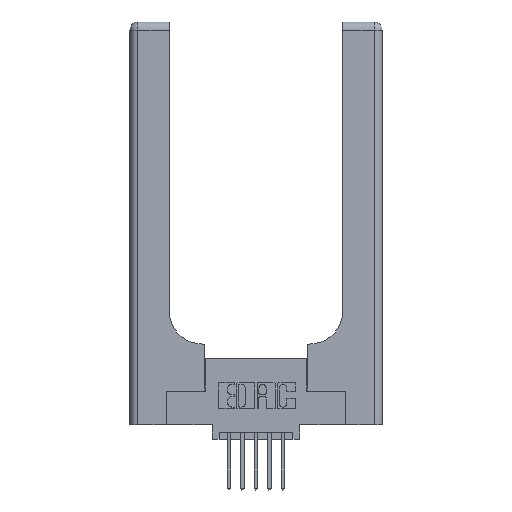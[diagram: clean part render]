
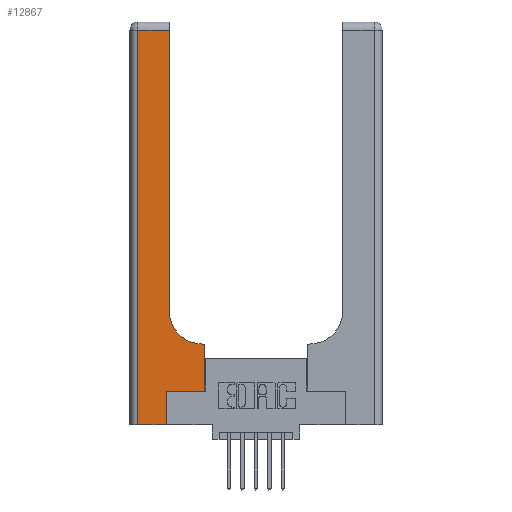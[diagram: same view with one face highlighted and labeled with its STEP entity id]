
A CAD part, top view. The second image highlights one B-rep face of the part: STEP entity #12867.
In plain terms, the highlighted planar face has unit normal (0, 0, 1).
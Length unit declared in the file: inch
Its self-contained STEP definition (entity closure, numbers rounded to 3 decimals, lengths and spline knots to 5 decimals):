
#26 = ORIENTED_EDGE ( 'NONE', *, *, #11161, .T. ) ;
#106 = LINE ( 'NONE', #4159, #10593 ) ;
#375 = AXIS2_PLACEMENT_3D ( 'NONE', #1722, #13631, #4002 ) ;
#578 = DIRECTION ( 'NONE',  ( 0., 1., 0. ) ) ;
#934 = DIRECTION ( 'NONE',  ( 1., 0., 0. ) ) ;
#1104 = CARTESIAN_POINT ( 'NONE',  ( 0.2915, 2.94, 0.37 ) ) ;
#1150 = DIRECTION ( 'NONE',  ( 1., 0., 0. ) ) ;
#1170 = VECTOR ( 'NONE', #11558, 39.37008 ) ;
#1261 = VECTOR ( 'NONE', #10786, 39.37008 ) ;
#1339 = EDGE_CURVE ( 'NONE', #5536, #8725, #9312, .T. ) ;
#1435 = VERTEX_POINT ( 'NONE', #13698 ) ;
#1722 = CARTESIAN_POINT ( 'NONE',  ( 0., 3., 0.37 ) ) ;
#1921 = VERTEX_POINT ( 'NONE', #12745 ) ;
#2453 = EDGE_LOOP ( 'NONE', ( #26, #9946, #4429, #8226, #8557, #7320, #3724, #13202, #9207 ) ) ;
#2532 = CARTESIAN_POINT ( 'NONE',  ( 0.06, 0., 0.37 ) ) ;
#2547 = CIRCLE ( 'NONE', #4182, 0.25 ) ;
#2641 = DIRECTION ( 'NONE',  ( 1., 0., 0. ) ) ;
#2884 = PLANE ( 'NONE',  #375 ) ;
#3232 = VECTOR ( 'NONE', #6166, 39.37008 ) ;
#3325 = LINE ( 'NONE', #11666, #5566 ) ;
#3569 = LINE ( 'NONE', #4010, #3232 ) ;
#3589 = LINE ( 'NONE', #5410, #1261 ) ;
#3724 = ORIENTED_EDGE ( 'NONE', *, *, #6920, .T. ) ;
#3893 = CARTESIAN_POINT ( 'NONE',  ( 0.2915, 0.85, 0.37 ) ) ;
#4002 = DIRECTION ( 'NONE',  ( -1., 0., 0. ) ) ;
#4010 = CARTESIAN_POINT ( 'NONE',  ( 0.2915, 3., 0.37 ) ) ;
#4159 = CARTESIAN_POINT ( 'NONE',  ( 0.2915, 0.6, 0.37 ) ) ;
#4182 = AXIS2_PLACEMENT_3D ( 'NONE', #14233, #7846, #1150 ) ;
#4234 = VERTEX_POINT ( 'NONE', #3893 ) ;
#4429 = ORIENTED_EDGE ( 'NONE', *, *, #13873, .T. ) ;
#4535 = EDGE_CURVE ( 'NONE', #7372, #5585, #8105, .T. ) ;
#4775 = CARTESIAN_POINT ( 'NONE',  ( 0.06, 3., 0.37 ) ) ;
#4862 = CARTESIAN_POINT ( 'NONE',  ( 0.269, 0.25, 0.37 ) ) ;
#5177 = VECTOR ( 'NONE', #934, 39.37008 ) ;
#5410 = CARTESIAN_POINT ( 'NONE',  ( 0.269, 0., 0.37 ) ) ;
#5425 = EDGE_CURVE ( 'NONE', #5585, #1435, #3589, .T. ) ;
#5536 = VERTEX_POINT ( 'NONE', #1104 ) ;
#5565 = EDGE_CURVE ( 'NONE', #6140, #4234, #2547, .T. ) ;
#5566 = VECTOR ( 'NONE', #578, 39.37008 ) ;
#5585 = VERTEX_POINT ( 'NONE', #13233 ) ;
#6140 = VERTEX_POINT ( 'NONE', #7687 ) ;
#6166 = DIRECTION ( 'NONE',  ( 0., 1., 0. ) ) ;
#6612 = VECTOR ( 'NONE', #2641, 39.37008 ) ;
#6920 = EDGE_CURVE ( 'NONE', #1921, #7972, #3325, .T. ) ;
#6950 = LINE ( 'NONE', #4862, #6612 ) ;
#7320 = ORIENTED_EDGE ( 'NONE', *, *, #12747, .T. ) ;
#7372 = VERTEX_POINT ( 'NONE', #2532 ) ;
#7687 = CARTESIAN_POINT ( 'NONE',  ( 0.5415, 0.6, 0.37 ) ) ;
#7846 = DIRECTION ( 'NONE',  ( 0., 0., -1. ) ) ;
#7972 = VERTEX_POINT ( 'NONE', #11363 ) ;
#8105 = LINE ( 'NONE', #8712, #5177 ) ;
#8226 = ORIENTED_EDGE ( 'NONE', *, *, #4535, .T. ) ;
#8277 = FACE_OUTER_BOUND ( 'NONE', #2453, .T. ) ;
#8557 = ORIENTED_EDGE ( 'NONE', *, *, #5425, .T. ) ;
#8712 = CARTESIAN_POINT ( 'NONE',  ( 0., 0., 0.37 ) ) ;
#8725 = VERTEX_POINT ( 'NONE', #9721 ) ;
#9207 = ORIENTED_EDGE ( 'NONE', *, *, #5565, .T. ) ;
#9312 = LINE ( 'NONE', #13678, #1170 ) ;
#9721 = CARTESIAN_POINT ( 'NONE',  ( 0.06, 2.94, 0.37 ) ) ;
#9946 = ORIENTED_EDGE ( 'NONE', *, *, #1339, .T. ) ;
#10593 = VECTOR ( 'NONE', #12820, 39.37008 ) ;
#10780 = LINE ( 'NONE', #4775, #13583 ) ;
#10786 = DIRECTION ( 'NONE',  ( 0., 1., 0. ) ) ;
#11161 = EDGE_CURVE ( 'NONE', #4234, #5536, #3569, .T. ) ;
#11239 = EDGE_CURVE ( 'NONE', #7972, #6140, #106, .T. ) ;
#11317 = DIRECTION ( 'NONE',  ( 0., -1., 0. ) ) ;
#11363 = CARTESIAN_POINT ( 'NONE',  ( 0.5585, 0.6, 0.37 ) ) ;
#11558 = DIRECTION ( 'NONE',  ( -1., 0., 0. ) ) ;
#11666 = CARTESIAN_POINT ( 'NONE',  ( 0.5585, 0.25, 0.37 ) ) ;
#12745 = CARTESIAN_POINT ( 'NONE',  ( 0.5585, 0.25, 0.37 ) ) ;
#12747 = EDGE_CURVE ( 'NONE', #1435, #1921, #6950, .T. ) ;
#12820 = DIRECTION ( 'NONE',  ( -1., 0., 0. ) ) ;
#12867 = ADVANCED_FACE ( 'NONE', ( #8277 ), #2884, .F. ) ;
#13202 = ORIENTED_EDGE ( 'NONE', *, *, #11239, .T. ) ;
#13233 = CARTESIAN_POINT ( 'NONE',  ( 0.269, 0., 0.37 ) ) ;
#13583 = VECTOR ( 'NONE', #11317, 39.37008 ) ;
#13631 = DIRECTION ( 'NONE',  ( 0., 0., -1. ) ) ;
#13678 = CARTESIAN_POINT ( 'NONE',  ( 0., 2.94, 0.37 ) ) ;
#13698 = CARTESIAN_POINT ( 'NONE',  ( 0.269, 0.25, 0.37 ) ) ;
#13873 = EDGE_CURVE ( 'NONE', #8725, #7372, #10780, .T. ) ;
#14233 = CARTESIAN_POINT ( 'NONE',  ( 0.5415, 0.85, 0.37 ) ) ;
